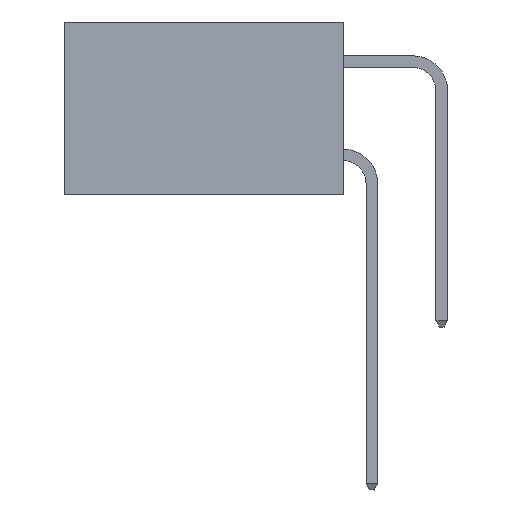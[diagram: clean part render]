
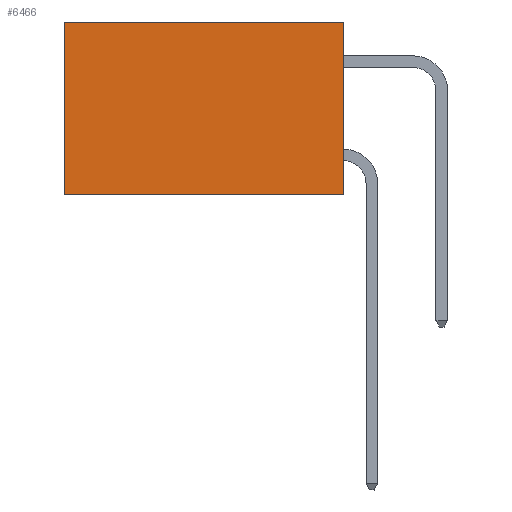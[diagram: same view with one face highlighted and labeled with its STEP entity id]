
A CAD part, left-side view. The second image highlights one B-rep face of the part: STEP entity #6466.
In plain terms, the highlighted planar face has unit normal (-1, 0, 0).
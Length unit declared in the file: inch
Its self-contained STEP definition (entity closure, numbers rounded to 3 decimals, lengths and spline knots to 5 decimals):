
#442 = VERTEX_POINT ( 'NONE', #4494 ) ;
#807 = CARTESIAN_POINT ( 'NONE',  ( 0.2615, 0., -0.37 ) ) ;
#1774 = CARTESIAN_POINT ( 'NONE',  ( 0.2615, 0., -0.37 ) ) ;
#1823 = LINE ( 'NONE', #14312, #5026 ) ;
#3076 = DIRECTION ( 'NONE',  ( 0., 1., 0. ) ) ;
#3143 = VECTOR ( 'NONE', #3165, 39.37008 ) ;
#3165 = DIRECTION ( 'NONE',  ( 0., 0., -1. ) ) ;
#3406 = DIRECTION ( 'NONE',  ( 0., 0., -1. ) ) ;
#4046 = VERTEX_POINT ( 'NONE', #807 ) ;
#4167 = PLANE ( 'NONE',  #13361 ) ;
#4494 = CARTESIAN_POINT ( 'NONE',  ( 0.2615, 0.6, -0.37 ) ) ;
#5026 = VECTOR ( 'NONE', #3076, 39.37008 ) ;
#5088 = EDGE_CURVE ( 'NONE', #4046, #442, #13161, .T. ) ;
#5643 = DIRECTION ( 'NONE',  ( 0., 0., -1. ) ) ;
#6466 = ADVANCED_FACE ( 'NONE', ( #14947 ), #4167, .F. ) ;
#6616 = LINE ( 'NONE', #15387, #3143 ) ;
#7562 = VECTOR ( 'NONE', #15791, 39.37008 ) ;
#8201 = EDGE_CURVE ( 'NONE', #9051, #4046, #6616, .T. ) ;
#9051 = VERTEX_POINT ( 'NONE', #11567 ) ;
#9099 = DIRECTION ( 'NONE',  ( 1., 0., 0. ) ) ;
#10162 = EDGE_CURVE ( 'NONE', #13731, #442, #13069, .T. ) ;
#10171 = EDGE_CURVE ( 'NONE', #9051, #13731, #1823, .T. ) ;
#10713 = EDGE_LOOP ( 'NONE', ( #14501, #13979, #14717, #15573 ) ) ;
#11567 = CARTESIAN_POINT ( 'NONE',  ( 0.2615, 0., 0. ) ) ;
#11832 = VECTOR ( 'NONE', #3406, 39.37008 ) ;
#13069 = LINE ( 'NONE', #15542, #11832 ) ;
#13074 = CARTESIAN_POINT ( 'NONE',  ( 0.2615, 0., -0.37 ) ) ;
#13161 = LINE ( 'NONE', #13074, #7562 ) ;
#13361 = AXIS2_PLACEMENT_3D ( 'NONE', #1774, #9099, #5643 ) ;
#13731 = VERTEX_POINT ( 'NONE', #15908 ) ;
#13979 = ORIENTED_EDGE ( 'NONE', *, *, #5088, .F. ) ;
#14312 = CARTESIAN_POINT ( 'NONE',  ( 0.2615, 0., 0. ) ) ;
#14501 = ORIENTED_EDGE ( 'NONE', *, *, #10162, .T. ) ;
#14717 = ORIENTED_EDGE ( 'NONE', *, *, #8201, .F. ) ;
#14947 = FACE_OUTER_BOUND ( 'NONE', #10713, .T. ) ;
#15387 = CARTESIAN_POINT ( 'NONE',  ( 0.2615, 0., -0.37 ) ) ;
#15542 = CARTESIAN_POINT ( 'NONE',  ( 0.2615, 0.6, -0.37 ) ) ;
#15573 = ORIENTED_EDGE ( 'NONE', *, *, #10171, .T. ) ;
#15791 = DIRECTION ( 'NONE',  ( 0., 1., 0. ) ) ;
#15908 = CARTESIAN_POINT ( 'NONE',  ( 0.2615, 0.6, 0. ) ) ;
